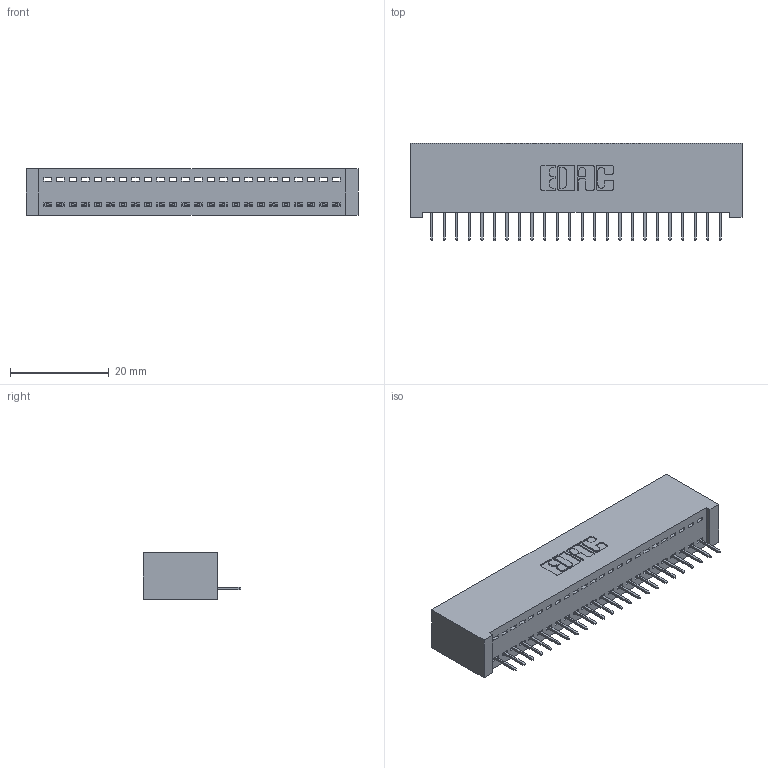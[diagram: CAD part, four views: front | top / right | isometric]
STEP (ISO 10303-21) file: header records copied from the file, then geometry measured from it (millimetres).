
FILE_DESCRIPTION (( 'STEP AP203' ), '1' );
FILE_NAME ('342-024-524-101.STEP', '2018-08-11T02:15:24', ( '' ), ( '' ), 'SwSTEP 2.0', 'SolidWorks 2016', '' );
FILE_SCHEMA (( 'CONFIG_CONTROL_DESIGN' ));
Length unit declared in the file: inch
Products named in the file (3): 345-292-001_345-293-124; 342-024-524-101; 342 Part_Lugless
Assembly tree (25 placements, depth 2):
  342-024-524-101
    342 Part_Lugless
    345-292-001_345-293-124  x24
Bounding box: 67.21 x 19.69 x 9.4 mm (x, y, z)
Volume: 6140.7 mm3; surface area: 8710.1 mm2
Topology: 25 solids, 25 shells, 1590 faces, 4595 edges, 2966 vertices
Faces by surface type: plane 1214, cylinder 376
Entity records: 16665 total; most frequent: CARTESIAN_POINT 2882, ORIENTED_EDGE 2842, DIRECTION 2461, EDGE_CURVE 1421, VECTOR 1305, LINE 1305, VERTEX_POINT 942, AXIS2_PLACEMENT_3D 578
